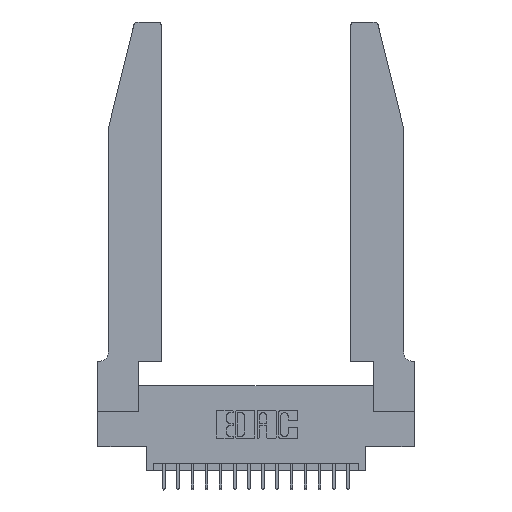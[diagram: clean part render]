
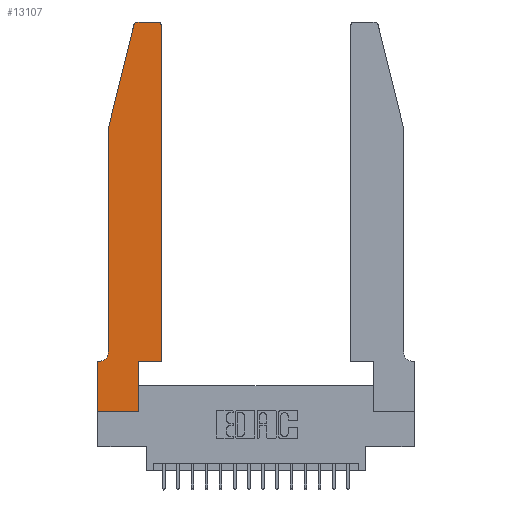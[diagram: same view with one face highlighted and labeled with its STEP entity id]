
A CAD part, top view. The second image highlights one B-rep face of the part: STEP entity #13107.
In plain terms, the highlighted planar face has unit normal (0, 0, 1).
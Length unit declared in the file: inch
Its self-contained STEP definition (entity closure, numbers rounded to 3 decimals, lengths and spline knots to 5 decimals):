
#6 = LINE ( 'NONE', #3026, #11032 ) ;
#154 = VECTOR ( 'NONE', #1328, 39.37008 ) ;
#727 = DIRECTION ( 'NONE',  ( 0., 0., 1. ) ) ;
#850 = CARTESIAN_POINT ( 'NONE',  ( 0., 0.35, 0.37 ) ) ;
#927 = CARTESIAN_POINT ( 'NONE',  ( 0.4205, 2.72, 0.37 ) ) ;
#1011 = DIRECTION ( 'NONE',  ( 1., 0., 0. ) ) ;
#1135 = EDGE_CURVE ( 'NONE', #8777, #13311, #17728, .T. ) ;
#1328 = DIRECTION ( 'NONE',  ( 0., 1., 0. ) ) ;
#1332 = ORIENTED_EDGE ( 'NONE', *, *, #18100, .T. ) ;
#1894 = DIRECTION ( 'NONE',  ( -1., 0., 0. ) ) ;
#2301 = VECTOR ( 'NONE', #8412, 39.37008 ) ;
#2463 = PLANE ( 'NONE',  #3920 ) ;
#2586 = VECTOR ( 'NONE', #17851, 39.37008 ) ;
#2959 = DIRECTION ( 'NONE',  ( 0., -1., 0. ) ) ;
#3026 = CARTESIAN_POINT ( 'NONE',  ( 0.0755, 0.35, 0.37 ) ) ;
#3324 = CARTESIAN_POINT ( 'NONE',  ( 0., 0., 0.37 ) ) ;
#3660 = ORIENTED_EDGE ( 'NONE', *, *, #18841, .T. ) ;
#3920 = AXIS2_PLACEMENT_3D ( 'NONE', #850, #10226, #17521 ) ;
#4072 = DIRECTION ( 'NONE',  ( 0., 1., 0. ) ) ;
#4077 = ORIENTED_EDGE ( 'NONE', *, *, #5300, .T. ) ;
#4167 = VECTOR ( 'NONE', #4072, 39.37008 ) ;
#4454 = ORIENTED_EDGE ( 'NONE', *, *, #6772, .T. ) ;
#5300 = EDGE_CURVE ( 'NONE', #11915, #12265, #11749, .T. ) ;
#5944 = LINE ( 'NONE', #12017, #7222 ) ;
#5982 = DIRECTION ( 'NONE',  ( 1., 0., 0. ) ) ;
#6361 = ORIENTED_EDGE ( 'NONE', *, *, #10803, .T. ) ;
#6579 = VECTOR ( 'NONE', #7307, 39.37008 ) ;
#6772 = EDGE_CURVE ( 'NONE', #7597, #8777, #10180, .T. ) ;
#6877 = AXIS2_PLACEMENT_3D ( 'NONE', #927, #7041, #13101 ) ;
#6924 = CARTESIAN_POINT ( 'NONE',  ( 0.0755, 2., 0.37 ) ) ;
#7041 = DIRECTION ( 'NONE',  ( 0., 0., 1. ) ) ;
#7077 = CARTESIAN_POINT ( 'NONE',  ( 0., 0., 0.37 ) ) ;
#7205 = CARTESIAN_POINT ( 'NONE',  ( 0.2865, 0.35, 0.37 ) ) ;
#7212 = ORIENTED_EDGE ( 'NONE', *, *, #7641, .T. ) ;
#7222 = VECTOR ( 'NONE', #2959, 39.37008 ) ;
#7307 = DIRECTION ( 'NONE',  ( -0.239, -0.971, 0. ) ) ;
#7597 = VERTEX_POINT ( 'NONE', #8504 ) ;
#7641 = EDGE_CURVE ( 'NONE', #8031, #9216, #10414, .T. ) ;
#8031 = VERTEX_POINT ( 'NONE', #7205 ) ;
#8187 = ORIENTED_EDGE ( 'NONE', *, *, #14956, .T. ) ;
#8412 = DIRECTION ( 'NONE',  ( 1., 0., 0. ) ) ;
#8480 = CARTESIAN_POINT ( 'NONE',  ( 0., 0., 0.37 ) ) ;
#8504 = CARTESIAN_POINT ( 'NONE',  ( 0., 0.35, 0.37 ) ) ;
#8777 = VERTEX_POINT ( 'NONE', #3324 ) ;
#8783 = EDGE_CURVE ( 'NONE', #10123, #18695, #9948, .T. ) ;
#8823 = CARTESIAN_POINT ( 'NONE',  ( 0.0055, 0.35, 0.37 ) ) ;
#9000 = DIRECTION ( 'NONE',  ( -1., 0., 0. ) ) ;
#9215 = AXIS2_PLACEMENT_3D ( 'NONE', #11798, #727, #1011 ) ;
#9216 = VERTEX_POINT ( 'NONE', #9576 ) ;
#9426 = CIRCLE ( 'NONE', #6877, 0.03 ) ;
#9483 = CARTESIAN_POINT ( 'NONE',  ( 0.284, 2.75, 0.37 ) ) ;
#9576 = CARTESIAN_POINT ( 'NONE',  ( 0.4505, 0.35, 0.37 ) ) ;
#9793 = DIRECTION ( 'NONE',  ( -1., 0., 0. ) ) ;
#9948 = CIRCLE ( 'NONE', #17583, 0.07 ) ;
#10123 = VERTEX_POINT ( 'NONE', #13701 ) ;
#10180 = LINE ( 'NONE', #8480, #2586 ) ;
#10226 = DIRECTION ( 'NONE',  ( 0., 0., 1. ) ) ;
#10403 = CARTESIAN_POINT ( 'NONE',  ( 0.4205, 2.75, 0.37 ) ) ;
#10414 = LINE ( 'NONE', #16499, #2301 ) ;
#10418 = LINE ( 'NONE', #16817, #154 ) ;
#10548 = VERTEX_POINT ( 'NONE', #14955 ) ;
#10670 = LINE ( 'NONE', #12842, #11001 ) ;
#10803 = EDGE_CURVE ( 'NONE', #13311, #8031, #14731, .T. ) ;
#11001 = VECTOR ( 'NONE', #1894, 39.37008 ) ;
#11032 = VECTOR ( 'NONE', #9000, 39.37008 ) ;
#11749 = CIRCLE ( 'NONE', #9215, 0.03 ) ;
#11781 = ORIENTED_EDGE ( 'NONE', *, *, #18013, .T. ) ;
#11798 = CARTESIAN_POINT ( 'NONE',  ( 0.284, 2.72, 0.37 ) ) ;
#11915 = VERTEX_POINT ( 'NONE', #9483 ) ;
#12017 = CARTESIAN_POINT ( 'NONE',  ( 0.0755, 2., 0.37 ) ) ;
#12179 = ORIENTED_EDGE ( 'NONE', *, *, #1135, .T. ) ;
#12265 = VERTEX_POINT ( 'NONE', #18538 ) ;
#12591 = DIRECTION ( 'NONE',  ( 0., 0., -1. ) ) ;
#12842 = CARTESIAN_POINT ( 'NONE',  ( 0.2605, 2.75, 0.37 ) ) ;
#12945 = CARTESIAN_POINT ( 'NONE',  ( 0.2865, 0.35, 0.37 ) ) ;
#13101 = DIRECTION ( 'NONE',  ( 1., 0., 0. ) ) ;
#13107 = ADVANCED_FACE ( 'NONE', ( #16127 ), #2463, .T. ) ;
#13311 = VERTEX_POINT ( 'NONE', #15877 ) ;
#13701 = CARTESIAN_POINT ( 'NONE',  ( 0.0755, 0.42, 0.37 ) ) ;
#14731 = LINE ( 'NONE', #12945, #4167 ) ;
#14868 = EDGE_LOOP ( 'NONE', ( #14949, #4077, #1332, #3660, #15237, #11781, #4454, #12179, #6361, #7212, #8187, #15379 ) ) ;
#14949 = ORIENTED_EDGE ( 'NONE', *, *, #15382, .T. ) ;
#14955 = CARTESIAN_POINT ( 'NONE',  ( 0.4505, 2.72, 0.37 ) ) ;
#14956 = EDGE_CURVE ( 'NONE', #9216, #10548, #10418, .T. ) ;
#15237 = ORIENTED_EDGE ( 'NONE', *, *, #8783, .T. ) ;
#15379 = ORIENTED_EDGE ( 'NONE', *, *, #17615, .T. ) ;
#15382 = EDGE_CURVE ( 'NONE', #19375, #11915, #10670, .T. ) ;
#15486 = CARTESIAN_POINT ( 'NONE',  ( 0.0055, 0.42, 0.37 ) ) ;
#15877 = CARTESIAN_POINT ( 'NONE',  ( 0.2865, 0., 0.37 ) ) ;
#16127 = FACE_OUTER_BOUND ( 'NONE', #14868, .T. ) ;
#16493 = VERTEX_POINT ( 'NONE', #6924 ) ;
#16499 = CARTESIAN_POINT ( 'NONE',  ( 0.4505, 0.35, 0.37 ) ) ;
#16589 = CARTESIAN_POINT ( 'NONE',  ( 0.0755, 2., 0.37 ) ) ;
#16817 = CARTESIAN_POINT ( 'NONE',  ( 0.4505, 0.35, 0.37 ) ) ;
#17105 = VECTOR ( 'NONE', #5982, 39.37008 ) ;
#17521 = DIRECTION ( 'NONE',  ( 1., 0., 0. ) ) ;
#17583 = AXIS2_PLACEMENT_3D ( 'NONE', #15486, #12591, #9793 ) ;
#17615 = EDGE_CURVE ( 'NONE', #10548, #19375, #9426, .T. ) ;
#17728 = LINE ( 'NONE', #7077, #17105 ) ;
#17851 = DIRECTION ( 'NONE',  ( 0., -1., 0. ) ) ;
#18013 = EDGE_CURVE ( 'NONE', #18695, #7597, #6, .T. ) ;
#18073 = LINE ( 'NONE', #16589, #6579 ) ;
#18100 = EDGE_CURVE ( 'NONE', #12265, #16493, #18073, .T. ) ;
#18538 = CARTESIAN_POINT ( 'NONE',  ( 0.25487, 2.72718, 0.37 ) ) ;
#18695 = VERTEX_POINT ( 'NONE', #8823 ) ;
#18841 = EDGE_CURVE ( 'NONE', #16493, #10123, #5944, .T. ) ;
#19375 = VERTEX_POINT ( 'NONE', #10403 ) ;
